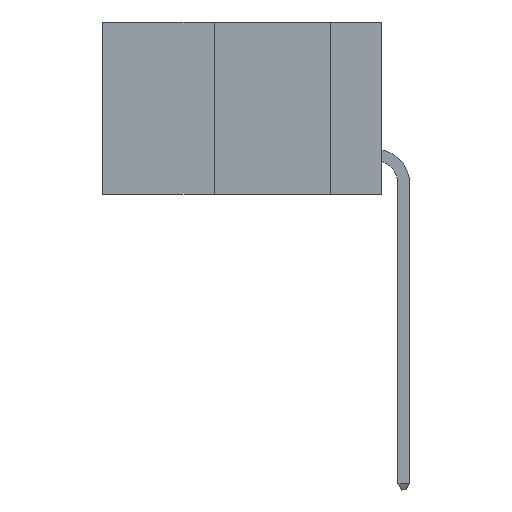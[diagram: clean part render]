
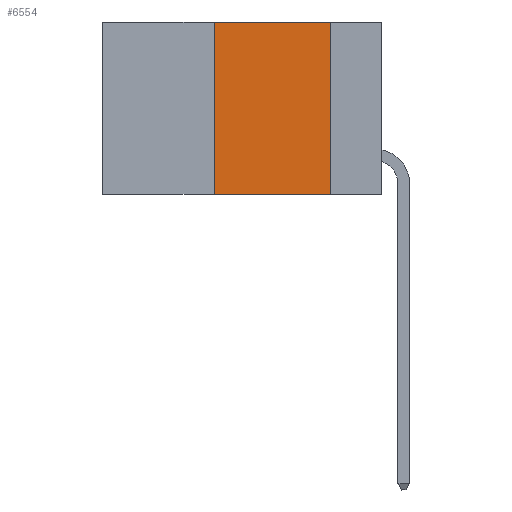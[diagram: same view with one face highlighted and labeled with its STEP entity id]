
A CAD part, left-side view. The second image highlights one B-rep face of the part: STEP entity #6554.
In plain terms, the highlighted planar face has unit normal (-1, 0, 0).
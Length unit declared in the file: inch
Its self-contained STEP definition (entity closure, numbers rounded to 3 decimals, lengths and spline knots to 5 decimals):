
#573 = CARTESIAN_POINT ( 'NONE',  ( 0., 0.11, 0. ) ) ;
#671 = DIRECTION ( 'NONE',  ( 0., 0., 1. ) ) ;
#1269 = VECTOR ( 'NONE', #15363, 39.37008 ) ;
#2027 = LINE ( 'NONE', #17906, #2466 ) ;
#2466 = VECTOR ( 'NONE', #671, 39.37008 ) ;
#2914 = CARTESIAN_POINT ( 'NONE',  ( 0., 0.11, 0. ) ) ;
#3413 = FACE_OUTER_BOUND ( 'NONE', #18471, .T. ) ;
#3515 = PLANE ( 'NONE',  #19609 ) ;
#3891 = ORIENTED_EDGE ( 'NONE', *, *, #16282, .F. ) ;
#4455 = CARTESIAN_POINT ( 'NONE',  ( 0., 0.6, -0.37 ) ) ;
#4828 = EDGE_CURVE ( 'NONE', #15197, #17199, #11011, .T. ) ;
#5068 = DIRECTION ( 'NONE',  ( 1., 0., 0. ) ) ;
#5857 = EDGE_CURVE ( 'NONE', #11511, #16314, #15464, .T. ) ;
#6554 = ADVANCED_FACE ( 'NONE', ( #3413 ), #3515, .F. ) ;
#6983 = CARTESIAN_POINT ( 'NONE',  ( 0., 0.36, -0.37 ) ) ;
#7046 = ORIENTED_EDGE ( 'NONE', *, *, #15315, .F. ) ;
#9849 = DIRECTION ( 'NONE',  ( 0., 0., -1. ) ) ;
#10254 = CARTESIAN_POINT ( 'NONE',  ( 0., 0.11, -0.37 ) ) ;
#10311 = ORIENTED_EDGE ( 'NONE', *, *, #5857, .F. ) ;
#11011 = LINE ( 'NONE', #4455, #13243 ) ;
#11126 = LINE ( 'NONE', #2914, #14019 ) ;
#11511 = VERTEX_POINT ( 'NONE', #17912 ) ;
#13243 = VECTOR ( 'NONE', #17351, 39.37008 ) ;
#14019 = VECTOR ( 'NONE', #14133, 39.37008 ) ;
#14133 = DIRECTION ( 'NONE',  ( 0., 0., -1. ) ) ;
#14719 = CARTESIAN_POINT ( 'NONE',  ( 0., 0.6, 0. ) ) ;
#15197 = VERTEX_POINT ( 'NONE', #6983 ) ;
#15315 = EDGE_CURVE ( 'NONE', #16314, #17199, #11126, .T. ) ;
#15363 = DIRECTION ( 'NONE',  ( 0., -1., 0. ) ) ;
#15464 = LINE ( 'NONE', #19850, #1269 ) ;
#16282 = EDGE_CURVE ( 'NONE', #15197, #11511, #2027, .T. ) ;
#16314 = VERTEX_POINT ( 'NONE', #573 ) ;
#17199 = VERTEX_POINT ( 'NONE', #10254 ) ;
#17351 = DIRECTION ( 'NONE',  ( 0., -1., 0. ) ) ;
#17906 = CARTESIAN_POINT ( 'NONE',  ( 0., 0.36, 0. ) ) ;
#17912 = CARTESIAN_POINT ( 'NONE',  ( 0., 0.36, 0. ) ) ;
#18471 = EDGE_LOOP ( 'NONE', ( #7046, #10311, #3891, #18814 ) ) ;
#18814 = ORIENTED_EDGE ( 'NONE', *, *, #4828, .T. ) ;
#19609 = AXIS2_PLACEMENT_3D ( 'NONE', #14719, #5068, #9849 ) ;
#19850 = CARTESIAN_POINT ( 'NONE',  ( 0., 0.6, 0. ) ) ;
